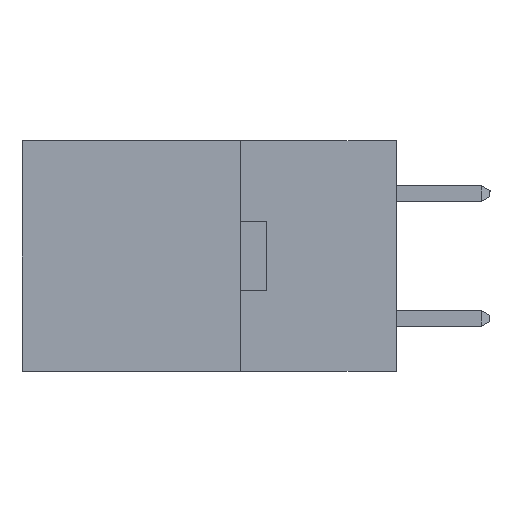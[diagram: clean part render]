
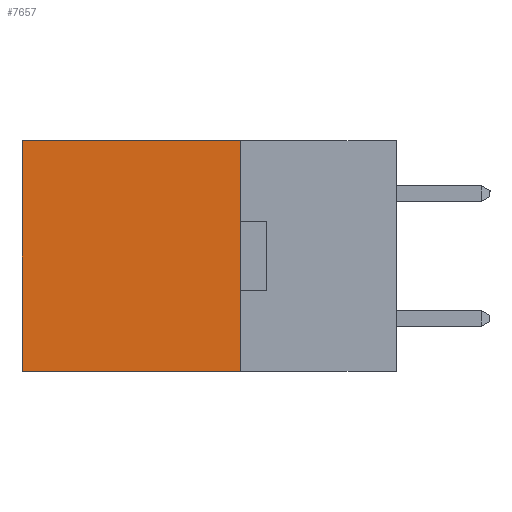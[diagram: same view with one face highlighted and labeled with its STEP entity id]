
A CAD part, left-side view. The second image highlights one B-rep face of the part: STEP entity #7657.
In plain terms, the highlighted planar face has unit normal (-1, 0, 0).
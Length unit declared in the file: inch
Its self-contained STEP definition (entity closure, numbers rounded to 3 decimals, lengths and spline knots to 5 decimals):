
#675 = DIRECTION ( 'NONE',  ( 0., 0., -1. ) ) ;
#772 = VECTOR ( 'NONE', #15852, 39.37008 ) ;
#2100 = VERTEX_POINT ( 'NONE', #20827 ) ;
#2114 = CARTESIAN_POINT ( 'NONE',  ( 0.2615, 0.25, -0.37 ) ) ;
#2397 = CARTESIAN_POINT ( 'NONE',  ( 0.2615, 0.6, -0.37 ) ) ;
#2830 = CARTESIAN_POINT ( 'NONE',  ( 0.2615, 0.25, -0.37 ) ) ;
#7617 = EDGE_CURVE ( 'NONE', #2100, #12670, #17845, .T. ) ;
#7657 = ADVANCED_FACE ( 'NONE', ( #13854 ), #22410, .F. ) ;
#8498 = CARTESIAN_POINT ( 'NONE',  ( 0.2615, 0.25, 0. ) ) ;
#8690 = LINE ( 'NONE', #12995, #12022 ) ;
#9265 = VERTEX_POINT ( 'NONE', #2114 ) ;
#10239 = EDGE_CURVE ( 'NONE', #9265, #12670, #14671, .T. ) ;
#10846 = LINE ( 'NONE', #23688, #13047 ) ;
#12022 = VECTOR ( 'NONE', #21705, 39.37008 ) ;
#12670 = VERTEX_POINT ( 'NONE', #20133 ) ;
#12836 = DIRECTION ( 'NONE',  ( 0., 0., -1. ) ) ;
#12995 = CARTESIAN_POINT ( 'NONE',  ( 0.2615, 0.25, 0. ) ) ;
#13047 = VECTOR ( 'NONE', #12836, 39.37008 ) ;
#13854 = FACE_OUTER_BOUND ( 'NONE', #22286, .T. ) ;
#14671 = LINE ( 'NONE', #14800, #26382 ) ;
#14800 = CARTESIAN_POINT ( 'NONE',  ( 0.2615, 0.25, -0.37 ) ) ;
#15852 = DIRECTION ( 'NONE',  ( 0., 0., -1. ) ) ;
#16364 = ORIENTED_EDGE ( 'NONE', *, *, #19954, .T. ) ;
#16571 = ORIENTED_EDGE ( 'NONE', *, *, #24409, .F. ) ;
#17845 = LINE ( 'NONE', #2397, #772 ) ;
#18281 = DIRECTION ( 'NONE',  ( 1., 0., 0. ) ) ;
#19714 = ORIENTED_EDGE ( 'NONE', *, *, #10239, .F. ) ;
#19954 = EDGE_CURVE ( 'NONE', #24919, #2100, #8690, .T. ) ;
#20133 = CARTESIAN_POINT ( 'NONE',  ( 0.2615, 0.6, -0.37 ) ) ;
#20827 = CARTESIAN_POINT ( 'NONE',  ( 0.2615, 0.6, 0. ) ) ;
#21705 = DIRECTION ( 'NONE',  ( 0., 1., 0. ) ) ;
#22286 = EDGE_LOOP ( 'NONE', ( #22628, #19714, #16571, #16364 ) ) ;
#22410 = PLANE ( 'NONE',  #25438 ) ;
#22628 = ORIENTED_EDGE ( 'NONE', *, *, #7617, .T. ) ;
#23688 = CARTESIAN_POINT ( 'NONE',  ( 0.2615, 0.25, -0.37 ) ) ;
#23766 = DIRECTION ( 'NONE',  ( 0., 1., 0. ) ) ;
#24409 = EDGE_CURVE ( 'NONE', #24919, #9265, #10846, .T. ) ;
#24919 = VERTEX_POINT ( 'NONE', #8498 ) ;
#25438 = AXIS2_PLACEMENT_3D ( 'NONE', #2830, #18281, #675 ) ;
#26382 = VECTOR ( 'NONE', #23766, 39.37008 ) ;
